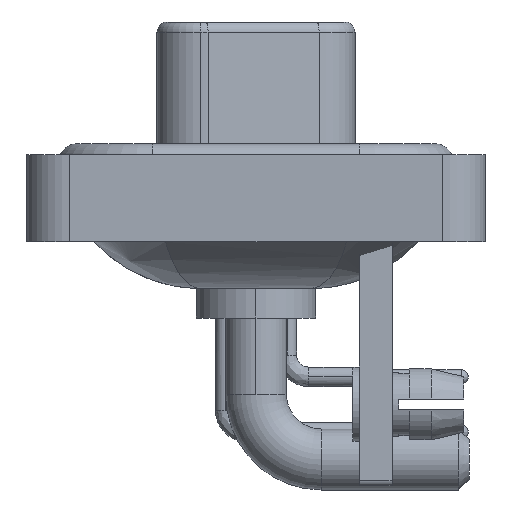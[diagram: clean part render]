
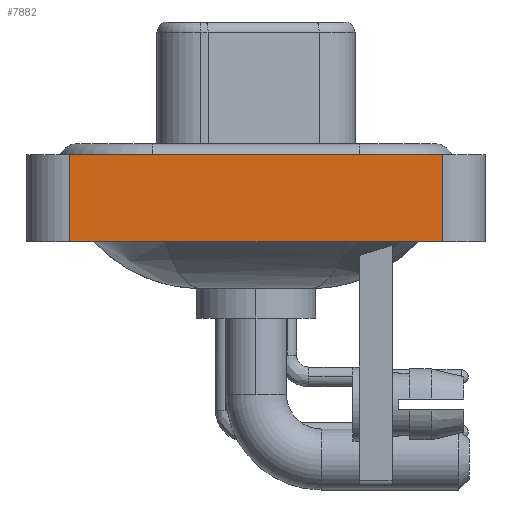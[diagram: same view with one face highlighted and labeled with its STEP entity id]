
A CAD part, left-side view. The second image highlights one B-rep face of the part: STEP entity #7882.
In plain terms, the highlighted planar face has unit normal (-1, 0, 0).
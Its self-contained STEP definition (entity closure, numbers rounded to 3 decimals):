
#89 = LINE ( 'NONE', #4159, #844 ) ;
#409 = VERTEX_POINT ( 'NONE', #13954 ) ;
#844 = VECTOR ( 'NONE', #25165, 1000. ) ;
#2339 = PLANE ( 'NONE',  #10948 ) ;
#3584 = DIRECTION ( 'NONE',  ( 0., 0., 1. ) ) ;
#4159 = CARTESIAN_POINT ( 'NONE',  ( -7.3, -8.55, -3.6 ) ) ;
#7882 = ADVANCED_FACE ( 'NONE', ( #12675 ), #2339, .T. ) ;
#8098 = CARTESIAN_POINT ( 'NONE',  ( -7.3, 8.55, 0.4 ) ) ;
#9380 = DIRECTION ( 'NONE',  ( 0., 0., 1. ) ) ;
#9648 = CARTESIAN_POINT ( 'NONE',  ( -7.3, -8.55, -3.6 ) ) ;
#9826 = VERTEX_POINT ( 'NONE', #22054 ) ;
#9968 = ORIENTED_EDGE ( 'NONE', *, *, #21694, .T. ) ;
#10103 = LINE ( 'NONE', #22256, #21255 ) ;
#10352 = VERTEX_POINT ( 'NONE', #16410 ) ;
#10835 = EDGE_CURVE ( 'NONE', #9826, #16730, #10103, .T. ) ;
#10948 = AXIS2_PLACEMENT_3D ( 'NONE', #23466, #13087, #15005 ) ;
#12675 = FACE_OUTER_BOUND ( 'NONE', #24715, .T. ) ;
#12817 = DIRECTION ( 'NONE',  ( 0., -1., 0. ) ) ;
#12912 = ORIENTED_EDGE ( 'NONE', *, *, #19879, .F. ) ;
#12957 = CARTESIAN_POINT ( 'NONE',  ( -7.3, -8.55, 0.4 ) ) ;
#13087 = DIRECTION ( 'NONE',  ( -1., 0., 0. ) ) ;
#13929 = VECTOR ( 'NONE', #12817, 1000. ) ;
#13954 = CARTESIAN_POINT ( 'NONE',  ( -7.3, -8.55, -3.6 ) ) ;
#15005 = DIRECTION ( 'NONE',  ( 0., 0., 1. ) ) ;
#15249 = ORIENTED_EDGE ( 'NONE', *, *, #10835, .F. ) ;
#16410 = CARTESIAN_POINT ( 'NONE',  ( -7.3, -8.55, 0.4 ) ) ;
#16730 = VERTEX_POINT ( 'NONE', #8098 ) ;
#16854 = EDGE_CURVE ( 'NONE', #9826, #409, #89, .T. ) ;
#17038 = LINE ( 'NONE', #12957, #13929 ) ;
#17956 = LINE ( 'NONE', #9648, #20237 ) ;
#19879 = EDGE_CURVE ( 'NONE', #16730, #10352, #17038, .T. ) ;
#20237 = VECTOR ( 'NONE', #9380, 1000. ) ;
#21255 = VECTOR ( 'NONE', #3584, 1000. ) ;
#21694 = EDGE_CURVE ( 'NONE', #409, #10352, #17956, .T. ) ;
#22054 = CARTESIAN_POINT ( 'NONE',  ( -7.3, 8.55, -3.6 ) ) ;
#22256 = CARTESIAN_POINT ( 'NONE',  ( -7.3, 8.55, -3.6 ) ) ;
#23466 = CARTESIAN_POINT ( 'NONE',  ( -7.3, -8.55, -3.6 ) ) ;
#24715 = EDGE_LOOP ( 'NONE', ( #9968, #12912, #15249, #26347 ) ) ;
#25165 = DIRECTION ( 'NONE',  ( 0., -1., 0. ) ) ;
#26347 = ORIENTED_EDGE ( 'NONE', *, *, #16854, .T. ) ;
